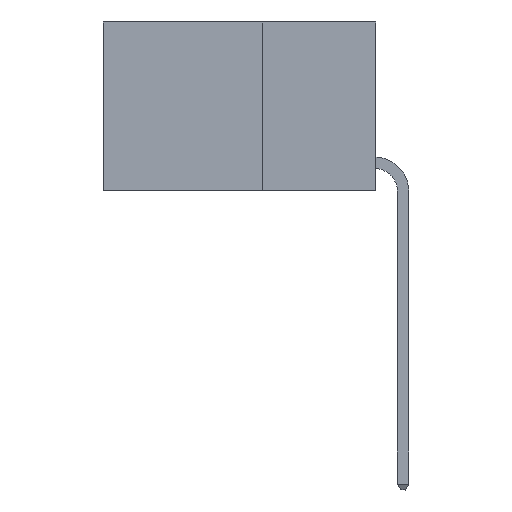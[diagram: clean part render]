
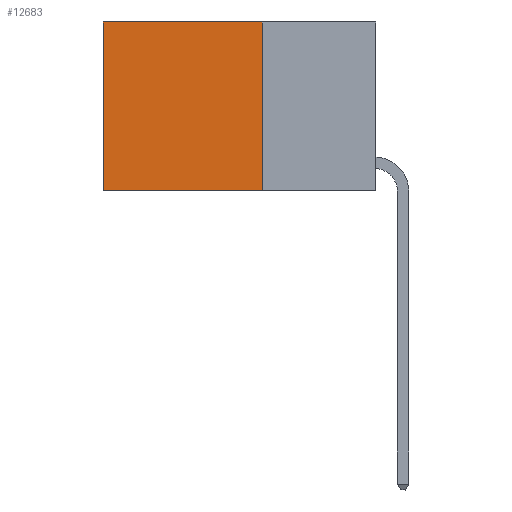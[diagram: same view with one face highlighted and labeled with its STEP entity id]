
A CAD part, left-side view. The second image highlights one B-rep face of the part: STEP entity #12683.
In plain terms, the highlighted planar face has unit normal (-1, 0, 0).
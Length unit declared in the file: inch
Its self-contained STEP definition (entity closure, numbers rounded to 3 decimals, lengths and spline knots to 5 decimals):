
#1069 = VECTOR ( 'NONE', #18202, 39.37008 ) ;
#2601 = VERTEX_POINT ( 'NONE', #14181 ) ;
#2827 = VERTEX_POINT ( 'NONE', #15088 ) ;
#3354 = ORIENTED_EDGE ( 'NONE', *, *, #15222, .T. ) ;
#4147 = ORIENTED_EDGE ( 'NONE', *, *, #16042, .T. ) ;
#4199 = ORIENTED_EDGE ( 'NONE', *, *, #10903, .F. ) ;
#5360 = LINE ( 'NONE', #16583, #1069 ) ;
#5609 = CARTESIAN_POINT ( 'NONE',  ( 0.2625, 0.25, -0.37 ) ) ;
#7179 = LINE ( 'NONE', #15513, #19475 ) ;
#9051 = DIRECTION ( 'NONE',  ( 0., 0., -1. ) ) ;
#9895 = DIRECTION ( 'NONE',  ( 0., 1., 0. ) ) ;
#10472 = VERTEX_POINT ( 'NONE', #13503 ) ;
#10603 = PLANE ( 'NONE',  #17526 ) ;
#10903 = EDGE_CURVE ( 'NONE', #10472, #17174, #5360, .T. ) ;
#10951 = EDGE_LOOP ( 'NONE', ( #3354, #16261, #4199, #4147 ) ) ;
#11419 = LINE ( 'NONE', #19471, #15674 ) ;
#12683 = ADVANCED_FACE ( 'NONE', ( #20334 ), #10603, .F. ) ;
#12706 = VECTOR ( 'NONE', #20054, 39.37008 ) ;
#13503 = CARTESIAN_POINT ( 'NONE',  ( 0.2625, 0.25, 0. ) ) ;
#14181 = CARTESIAN_POINT ( 'NONE',  ( 0.2625, 0.6, -0.37 ) ) ;
#15088 = CARTESIAN_POINT ( 'NONE',  ( 0.2625, 0.6, 0. ) ) ;
#15222 = EDGE_CURVE ( 'NONE', #2827, #2601, #7179, .T. ) ;
#15513 = CARTESIAN_POINT ( 'NONE',  ( 0.2625, 0.6, 0. ) ) ;
#15674 = VECTOR ( 'NONE', #9895, 39.37008 ) ;
#16042 = EDGE_CURVE ( 'NONE', #10472, #2827, #11419, .T. ) ;
#16261 = ORIENTED_EDGE ( 'NONE', *, *, #19162, .F. ) ;
#16583 = CARTESIAN_POINT ( 'NONE',  ( 0.2625, 0.25, 0. ) ) ;
#16978 = LINE ( 'NONE', #5609, #12706 ) ;
#17030 = CARTESIAN_POINT ( 'NONE',  ( 0.2625, 0.25, 0. ) ) ;
#17174 = VERTEX_POINT ( 'NONE', #20802 ) ;
#17526 = AXIS2_PLACEMENT_3D ( 'NONE', #17030, #18638, #9051 ) ;
#18202 = DIRECTION ( 'NONE',  ( 0., 0., -1. ) ) ;
#18638 = DIRECTION ( 'NONE',  ( 1., 0., 0. ) ) ;
#19162 = EDGE_CURVE ( 'NONE', #17174, #2601, #16978, .T. ) ;
#19471 = CARTESIAN_POINT ( 'NONE',  ( 0.2625, 0.25, 0. ) ) ;
#19475 = VECTOR ( 'NONE', #20264, 39.37008 ) ;
#20054 = DIRECTION ( 'NONE',  ( 0., 1., 0. ) ) ;
#20264 = DIRECTION ( 'NONE',  ( 0., 0., -1. ) ) ;
#20334 = FACE_OUTER_BOUND ( 'NONE', #10951, .T. ) ;
#20802 = CARTESIAN_POINT ( 'NONE',  ( 0.2625, 0.25, -0.37 ) ) ;
